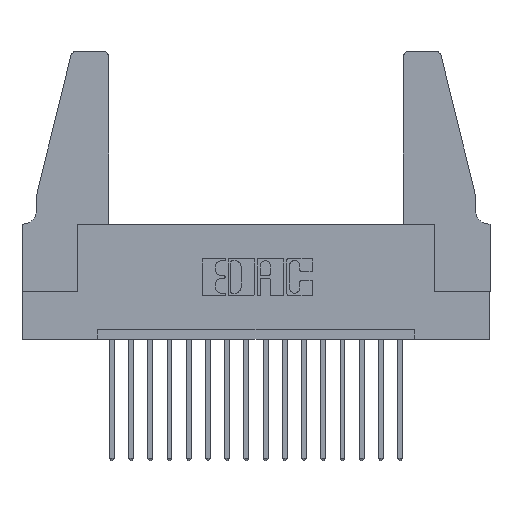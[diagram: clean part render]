
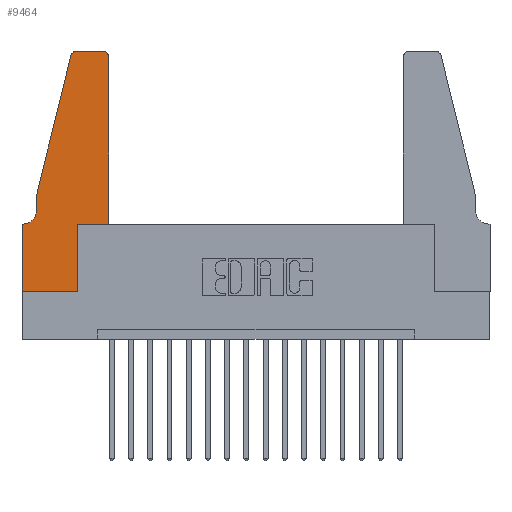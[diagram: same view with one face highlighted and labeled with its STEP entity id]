
A CAD part, top view. The second image highlights one B-rep face of the part: STEP entity #9464.
In plain terms, the highlighted planar face has unit normal (0, 0, 1).
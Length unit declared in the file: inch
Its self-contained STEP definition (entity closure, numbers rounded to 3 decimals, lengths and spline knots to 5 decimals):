
#192 = CARTESIAN_POINT ( 'NONE',  ( 0., 0., 0.37 ) ) ;
#502 = CARTESIAN_POINT ( 'NONE',  ( 0.0755, 0.42, 0.37 ) ) ;
#525 = CARTESIAN_POINT ( 'NONE',  ( 0., 0., 0.37 ) ) ;
#741 = CARTESIAN_POINT ( 'NONE',  ( 0.2865, 0., 0.37 ) ) ;
#1160 = FACE_OUTER_BOUND ( 'NONE', #11958, .T. ) ;
#1172 = LINE ( 'NONE', #15250, #11859 ) ;
#1291 = EDGE_CURVE ( 'NONE', #6709, #15705, #8358, .T. ) ;
#1705 = LINE ( 'NONE', #6830, #10687 ) ;
#1856 = ORIENTED_EDGE ( 'NONE', *, *, #8643, .T. ) ;
#1905 = DIRECTION ( 'NONE',  ( 1., 0., 0. ) ) ;
#2058 = VECTOR ( 'NONE', #6703, 39.37008 ) ;
#2129 = LINE ( 'NONE', #10329, #5531 ) ;
#2253 = CARTESIAN_POINT ( 'NONE',  ( 0., 0.35, 0.37 ) ) ;
#2326 = CARTESIAN_POINT ( 'NONE',  ( 0., 0.35, 0.37 ) ) ;
#2761 = VERTEX_POINT ( 'NONE', #741 ) ;
#2957 = DIRECTION ( 'NONE',  ( 0., -1., 0. ) ) ;
#3061 = DIRECTION ( 'NONE',  ( 0., 0., 1. ) ) ;
#3083 = EDGE_CURVE ( 'NONE', #11331, #17151, #1172, .T. ) ;
#3294 = CARTESIAN_POINT ( 'NONE',  ( 0.0755, 0.5, 0.37 ) ) ;
#3455 = EDGE_CURVE ( 'NONE', #5656, #3946, #5016, .T. ) ;
#3592 = LINE ( 'NONE', #9170, #13634 ) ;
#3604 = DIRECTION ( 'NONE',  ( 0., -1., 0. ) ) ;
#3655 = EDGE_CURVE ( 'NONE', #12991, #13132, #6099, .T. ) ;
#3669 = VERTEX_POINT ( 'NONE', #9660 ) ;
#3863 = CARTESIAN_POINT ( 'NONE',  ( 0.4205, 1.22, 0.37 ) ) ;
#3946 = VERTEX_POINT ( 'NONE', #8003 ) ;
#3992 = PLANE ( 'NONE',  #6520 ) ;
#3995 = EDGE_CURVE ( 'NONE', #3946, #5044, #11830, .T. ) ;
#4298 = ORIENTED_EDGE ( 'NONE', *, *, #6443, .T. ) ;
#4806 = LINE ( 'NONE', #15142, #2058 ) ;
#5016 = CIRCLE ( 'NONE', #13010, 0.03 ) ;
#5044 = VERTEX_POINT ( 'NONE', #3294 ) ;
#5323 = DIRECTION ( 'NONE',  ( -1., 0., 0. ) ) ;
#5531 = VECTOR ( 'NONE', #3604, 39.37008 ) ;
#5656 = VERTEX_POINT ( 'NONE', #9489 ) ;
#6099 = CIRCLE ( 'NONE', #16073, 0.03 ) ;
#6125 = DIRECTION ( 'NONE',  ( 1., 0., 0. ) ) ;
#6443 = EDGE_CURVE ( 'NONE', #5044, #6709, #2129, .T. ) ;
#6494 = DIRECTION ( 'NONE',  ( 0., 0., 1. ) ) ;
#6520 = AXIS2_PLACEMENT_3D ( 'NONE', #2326, #14516, #9025 ) ;
#6534 = CARTESIAN_POINT ( 'NONE',  ( 0.2865, 0.35, 0.37 ) ) ;
#6553 = DIRECTION ( 'NONE',  ( 1., 0., 0. ) ) ;
#6599 = EDGE_CURVE ( 'NONE', #17151, #2761, #17325, .T. ) ;
#6703 = DIRECTION ( 'NONE',  ( 0., 1., 0. ) ) ;
#6709 = VERTEX_POINT ( 'NONE', #502 ) ;
#6830 = CARTESIAN_POINT ( 'NONE',  ( 0.2605, 1.25, 0.37 ) ) ;
#6979 = DIRECTION ( 'NONE',  ( 1., 0., 0. ) ) ;
#7095 = CARTESIAN_POINT ( 'NONE',  ( 0.0755, 0.5, 0.37 ) ) ;
#7351 = EDGE_CURVE ( 'NONE', #15705, #11331, #3592, .T. ) ;
#7905 = ORIENTED_EDGE ( 'NONE', *, *, #12800, .T. ) ;
#8003 = CARTESIAN_POINT ( 'NONE',  ( 0.25487, 1.22718, 0.37 ) ) ;
#8253 = LINE ( 'NONE', #6534, #16804 ) ;
#8358 = CIRCLE ( 'NONE', #10452, 0.07 ) ;
#8453 = DIRECTION ( 'NONE',  ( 0., 0., -1. ) ) ;
#8576 = DIRECTION ( 'NONE',  ( -1., 0., 0. ) ) ;
#8643 = EDGE_CURVE ( 'NONE', #2761, #3669, #8253, .T. ) ;
#9025 = DIRECTION ( 'NONE',  ( 1., 0., 0. ) ) ;
#9159 = VERTEX_POINT ( 'NONE', #17692 ) ;
#9170 = CARTESIAN_POINT ( 'NONE',  ( 0.0755, 0.35, 0.37 ) ) ;
#9200 = VECTOR ( 'NONE', #1905, 39.37008 ) ;
#9464 = ADVANCED_FACE ( 'NONE', ( #1160 ), #3992, .T. ) ;
#9489 = CARTESIAN_POINT ( 'NONE',  ( 0.284, 1.25, 0.37 ) ) ;
#9629 = EDGE_CURVE ( 'NONE', #9159, #12991, #4806, .T. ) ;
#9660 = CARTESIAN_POINT ( 'NONE',  ( 0.2865, 0.35, 0.37 ) ) ;
#10329 = CARTESIAN_POINT ( 'NONE',  ( 0.0755, 0.5, 0.37 ) ) ;
#10452 = AXIS2_PLACEMENT_3D ( 'NONE', #15329, #8453, #8576 ) ;
#10559 = ORIENTED_EDGE ( 'NONE', *, *, #1291, .T. ) ;
#10662 = ORIENTED_EDGE ( 'NONE', *, *, #9629, .T. ) ;
#10687 = VECTOR ( 'NONE', #11017, 39.37008 ) ;
#11017 = DIRECTION ( 'NONE',  ( -1., 0., 0. ) ) ;
#11331 = VERTEX_POINT ( 'NONE', #2253 ) ;
#11830 = LINE ( 'NONE', #7095, #15467 ) ;
#11859 = VECTOR ( 'NONE', #2957, 39.37008 ) ;
#11958 = EDGE_LOOP ( 'NONE', ( #7905, #12437, #16226, #4298, #10559, #13576, #15135, #16403, #1856, #14535, #10662, #14816 ) ) ;
#12427 = DIRECTION ( 'NONE',  ( -0.239, -0.971, 0. ) ) ;
#12437 = ORIENTED_EDGE ( 'NONE', *, *, #3455, .T. ) ;
#12547 = EDGE_CURVE ( 'NONE', #3669, #9159, #16262, .T. ) ;
#12800 = EDGE_CURVE ( 'NONE', #13132, #5656, #1705, .T. ) ;
#12991 = VERTEX_POINT ( 'NONE', #16252 ) ;
#13010 = AXIS2_PLACEMENT_3D ( 'NONE', #13859, #3061, #6979 ) ;
#13132 = VERTEX_POINT ( 'NONE', #14907 ) ;
#13576 = ORIENTED_EDGE ( 'NONE', *, *, #7351, .T. ) ;
#13634 = VECTOR ( 'NONE', #5323, 39.37008 ) ;
#13859 = CARTESIAN_POINT ( 'NONE',  ( 0.284, 1.22, 0.37 ) ) ;
#13997 = CARTESIAN_POINT ( 'NONE',  ( 0.0055, 0.35, 0.37 ) ) ;
#14516 = DIRECTION ( 'NONE',  ( 0., 0., 1. ) ) ;
#14535 = ORIENTED_EDGE ( 'NONE', *, *, #12547, .T. ) ;
#14816 = ORIENTED_EDGE ( 'NONE', *, *, #3655, .T. ) ;
#14907 = CARTESIAN_POINT ( 'NONE',  ( 0.4205, 1.25, 0.37 ) ) ;
#15135 = ORIENTED_EDGE ( 'NONE', *, *, #3083, .T. ) ;
#15142 = CARTESIAN_POINT ( 'NONE',  ( 0.4505, 0.35, 0.37 ) ) ;
#15250 = CARTESIAN_POINT ( 'NONE',  ( 0., 0., 0.37 ) ) ;
#15329 = CARTESIAN_POINT ( 'NONE',  ( 0.0055, 0.42, 0.37 ) ) ;
#15467 = VECTOR ( 'NONE', #12427, 39.37008 ) ;
#15705 = VERTEX_POINT ( 'NONE', #13997 ) ;
#15862 = CARTESIAN_POINT ( 'NONE',  ( 0.4505, 0.35, 0.37 ) ) ;
#16073 = AXIS2_PLACEMENT_3D ( 'NONE', #3863, #6494, #6553 ) ;
#16226 = ORIENTED_EDGE ( 'NONE', *, *, #3995, .T. ) ;
#16252 = CARTESIAN_POINT ( 'NONE',  ( 0.4505, 1.22, 0.37 ) ) ;
#16262 = LINE ( 'NONE', #15862, #17574 ) ;
#16403 = ORIENTED_EDGE ( 'NONE', *, *, #6599, .T. ) ;
#16804 = VECTOR ( 'NONE', #17487, 39.37008 ) ;
#17151 = VERTEX_POINT ( 'NONE', #192 ) ;
#17325 = LINE ( 'NONE', #525, #9200 ) ;
#17487 = DIRECTION ( 'NONE',  ( 0., 1., 0. ) ) ;
#17574 = VECTOR ( 'NONE', #6125, 39.37008 ) ;
#17692 = CARTESIAN_POINT ( 'NONE',  ( 0.4505, 0.35, 0.37 ) ) ;
